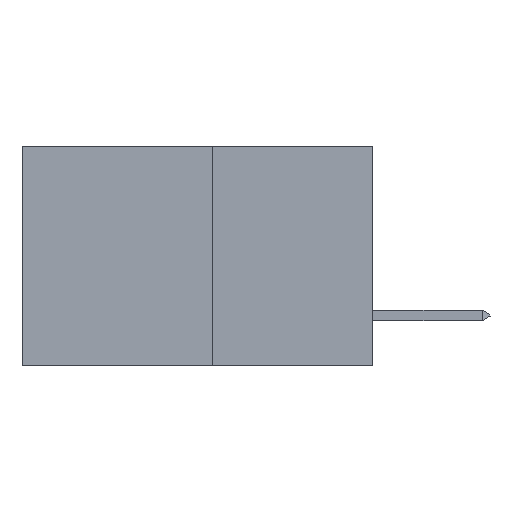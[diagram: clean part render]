
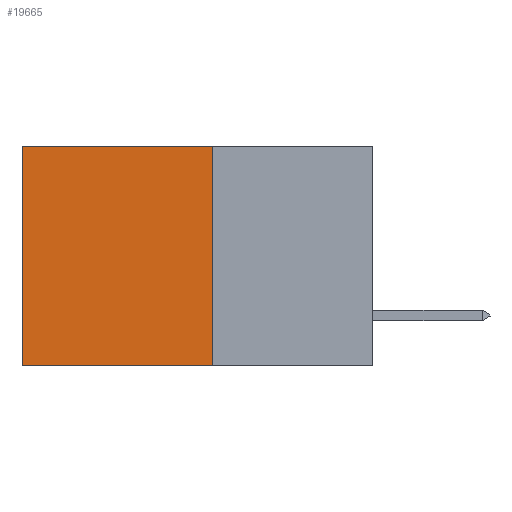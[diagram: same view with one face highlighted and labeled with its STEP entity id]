
A CAD part, left-side view. The second image highlights one B-rep face of the part: STEP entity #19665.
In plain terms, the highlighted planar face has unit normal (-1, 0, 0).
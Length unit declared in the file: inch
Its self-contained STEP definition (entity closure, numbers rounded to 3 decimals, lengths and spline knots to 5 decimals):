
#63 = DIRECTION ( 'NONE',  ( 0., 0., -1. ) ) ;
#72 = LINE ( 'NONE', #1902, #16325 ) ;
#1188 = PLANE ( 'NONE',  #18691 ) ;
#1357 = EDGE_CURVE ( 'NONE', #18513, #20221, #16424, .T. ) ;
#1407 = LINE ( 'NONE', #7915, #9240 ) ;
#1521 = CARTESIAN_POINT ( 'NONE',  ( 0.277, 0.59, -0.37 ) ) ;
#1729 = VERTEX_POINT ( 'NONE', #2246 ) ;
#1868 = FACE_OUTER_BOUND ( 'NONE', #19482, .T. ) ;
#1902 = CARTESIAN_POINT ( 'NONE',  ( 0.277, 0.59, -0.37 ) ) ;
#2049 = LINE ( 'NONE', #18790, #9870 ) ;
#2246 = CARTESIAN_POINT ( 'NONE',  ( 0.277, 0.27, -0.37 ) ) ;
#3436 = EDGE_CURVE ( 'NONE', #1729, #7280, #2049, .T. ) ;
#4381 = DIRECTION ( 'NONE',  ( 0., 0., -1. ) ) ;
#7280 = VERTEX_POINT ( 'NONE', #1521 ) ;
#7915 = CARTESIAN_POINT ( 'NONE',  ( 0.277, 0.27, -0.37 ) ) ;
#9112 = DIRECTION ( 'NONE',  ( 0., 1., 0. ) ) ;
#9240 = VECTOR ( 'NONE', #63, 39.37008 ) ;
#9756 = DIRECTION ( 'NONE',  ( 0., 0., -1. ) ) ;
#9870 = VECTOR ( 'NONE', #10500, 39.37008 ) ;
#10323 = CARTESIAN_POINT ( 'NONE',  ( 0.277, 0.59, 0. ) ) ;
#10500 = DIRECTION ( 'NONE',  ( 0., 1., 0. ) ) ;
#12201 = CARTESIAN_POINT ( 'NONE',  ( 0.277, 0.27, -0.37 ) ) ;
#12258 = VECTOR ( 'NONE', #9112, 39.37008 ) ;
#13803 = DIRECTION ( 'NONE',  ( 1., 0., 0. ) ) ;
#14422 = CARTESIAN_POINT ( 'NONE',  ( 0.277, 0.27, 0. ) ) ;
#15379 = ORIENTED_EDGE ( 'NONE', *, *, #3436, .F. ) ;
#16325 = VECTOR ( 'NONE', #9756, 39.37008 ) ;
#16424 = LINE ( 'NONE', #18679, #12258 ) ;
#16635 = ORIENTED_EDGE ( 'NONE', *, *, #1357, .T. ) ;
#17548 = ORIENTED_EDGE ( 'NONE', *, *, #19995, .T. ) ;
#18444 = EDGE_CURVE ( 'NONE', #18513, #1729, #1407, .T. ) ;
#18513 = VERTEX_POINT ( 'NONE', #14422 ) ;
#18679 = CARTESIAN_POINT ( 'NONE',  ( 0.277, 0.27, 0. ) ) ;
#18691 = AXIS2_PLACEMENT_3D ( 'NONE', #12201, #13803, #4381 ) ;
#18790 = CARTESIAN_POINT ( 'NONE',  ( 0.277, 0.27, -0.37 ) ) ;
#19482 = EDGE_LOOP ( 'NONE', ( #17548, #15379, #19513, #16635 ) ) ;
#19513 = ORIENTED_EDGE ( 'NONE', *, *, #18444, .F. ) ;
#19665 = ADVANCED_FACE ( 'NONE', ( #1868 ), #1188, .F. ) ;
#19995 = EDGE_CURVE ( 'NONE', #20221, #7280, #72, .T. ) ;
#20221 = VERTEX_POINT ( 'NONE', #10323 ) ;
